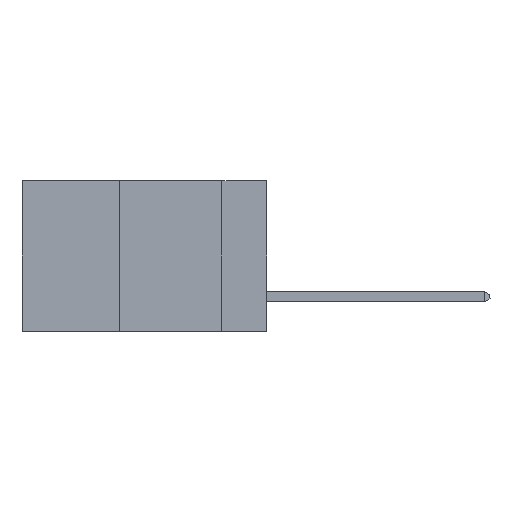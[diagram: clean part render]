
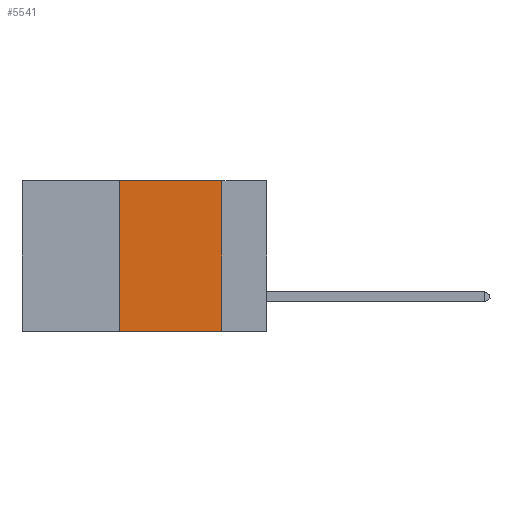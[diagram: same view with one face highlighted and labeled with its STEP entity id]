
A CAD part, left-side view. The second image highlights one B-rep face of the part: STEP entity #5541.
In plain terms, the highlighted planar face has unit normal (-1, 0, 0).
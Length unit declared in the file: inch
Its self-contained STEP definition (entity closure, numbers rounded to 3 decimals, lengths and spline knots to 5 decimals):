
#197 = VECTOR ( 'NONE', #4629, 39.37008 ) ;
#354 = ORIENTED_EDGE ( 'NONE', *, *, #11025, .F. ) ;
#510 = LINE ( 'NONE', #9626, #197 ) ;
#875 = LINE ( 'NONE', #12647, #1541 ) ;
#1064 = ORIENTED_EDGE ( 'NONE', *, *, #2358, .T. ) ;
#1541 = VECTOR ( 'NONE', #6900, 39.37008 ) ;
#1614 = CARTESIAN_POINT ( 'NONE',  ( 0., 0.36, -0.37 ) ) ;
#1707 = AXIS2_PLACEMENT_3D ( 'NONE', #4429, #4417, #4402 ) ;
#2090 = VERTEX_POINT ( 'NONE', #7749 ) ;
#2358 = EDGE_CURVE ( 'NONE', #9217, #6403, #4887, .T. ) ;
#2613 = EDGE_CURVE ( 'NONE', #9217, #2090, #7407, .T. ) ;
#4397 = VECTOR ( 'NONE', #8132, 39.37008 ) ;
#4402 = DIRECTION ( 'NONE',  ( 0., 0., -1. ) ) ;
#4417 = DIRECTION ( 'NONE',  ( 1., 0., 0. ) ) ;
#4429 = CARTESIAN_POINT ( 'NONE',  ( 0., 0.6, 0. ) ) ;
#4548 = PLANE ( 'NONE',  #1707 ) ;
#4629 = DIRECTION ( 'NONE',  ( 0., -1., 0. ) ) ;
#4887 = LINE ( 'NONE', #10781, #12802 ) ;
#5126 = EDGE_LOOP ( 'NONE', ( #354, #9867, #10056, #1064 ) ) ;
#5541 = ADVANCED_FACE ( 'NONE', ( #7077 ), #4548, .F. ) ;
#6147 = CARTESIAN_POINT ( 'NONE',  ( 0., 0.11, 0. ) ) ;
#6403 = VERTEX_POINT ( 'NONE', #12293 ) ;
#6560 = EDGE_CURVE ( 'NONE', #2090, #12005, #510, .T. ) ;
#6900 = DIRECTION ( 'NONE',  ( 0., 0., -1. ) ) ;
#7077 = FACE_OUTER_BOUND ( 'NONE', #5126, .T. ) ;
#7407 = LINE ( 'NONE', #8477, #4397 ) ;
#7749 = CARTESIAN_POINT ( 'NONE',  ( 0., 0.36, 0. ) ) ;
#8132 = DIRECTION ( 'NONE',  ( 0., 0., 1. ) ) ;
#8477 = CARTESIAN_POINT ( 'NONE',  ( 0., 0.36, 0. ) ) ;
#9217 = VERTEX_POINT ( 'NONE', #1614 ) ;
#9626 = CARTESIAN_POINT ( 'NONE',  ( 0., 0.6, 0. ) ) ;
#9867 = ORIENTED_EDGE ( 'NONE', *, *, #6560, .F. ) ;
#10056 = ORIENTED_EDGE ( 'NONE', *, *, #2613, .F. ) ;
#10778 = DIRECTION ( 'NONE',  ( 0., -1., 0. ) ) ;
#10781 = CARTESIAN_POINT ( 'NONE',  ( 0., 0.6, -0.37 ) ) ;
#11025 = EDGE_CURVE ( 'NONE', #12005, #6403, #875, .T. ) ;
#12005 = VERTEX_POINT ( 'NONE', #6147 ) ;
#12293 = CARTESIAN_POINT ( 'NONE',  ( 0., 0.11, -0.37 ) ) ;
#12647 = CARTESIAN_POINT ( 'NONE',  ( 0., 0.11, 0. ) ) ;
#12802 = VECTOR ( 'NONE', #10778, 39.37008 ) ;
